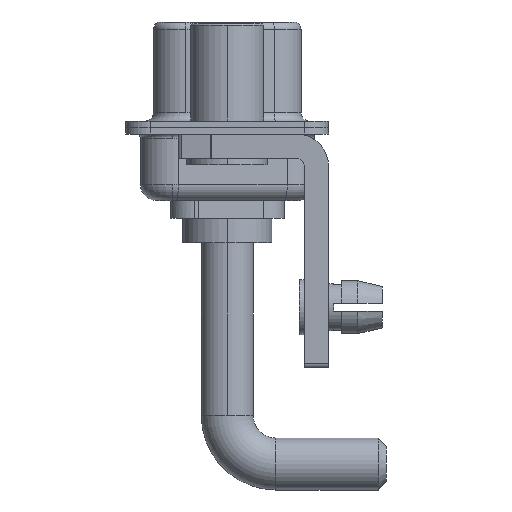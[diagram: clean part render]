
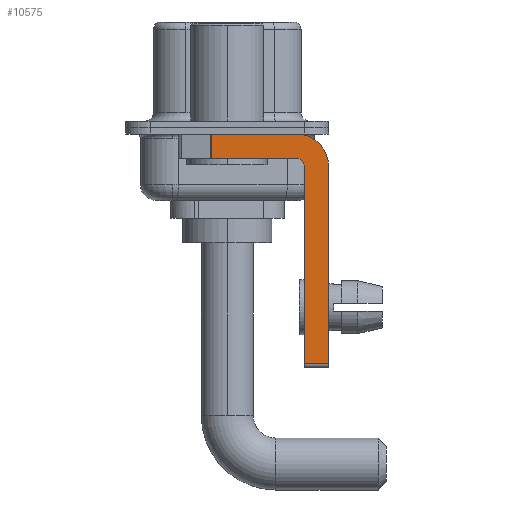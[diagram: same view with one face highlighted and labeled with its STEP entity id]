
A CAD part, left-side view. The second image highlights one B-rep face of the part: STEP entity #10575.
In plain terms, the highlighted planar face has unit normal (-1, 0, 0).
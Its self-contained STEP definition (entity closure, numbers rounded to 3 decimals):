
#59 = EDGE_CURVE ( 'NONE', #12031, #14969, #9710, .T. ) ;
#64 = LINE ( 'NONE', #1293, #7859 ) ;
#87 = DIRECTION ( 'NONE',  ( 0., 0., -1. ) ) ;
#227 = CARTESIAN_POINT ( 'NONE',  ( -2.9, -4.25, -2.4 ) ) ;
#367 = LINE ( 'NONE', #14322, #5056 ) ;
#567 = ORIENTED_EDGE ( 'NONE', *, *, #7969, .F. ) ;
#962 = CARTESIAN_POINT ( 'NONE',  ( -2.9, 0.978, -1.9 ) ) ;
#1140 = LINE ( 'NONE', #5623, #3806 ) ;
#1225 = ORIENTED_EDGE ( 'NONE', *, *, #59, .F. ) ;
#1293 = CARTESIAN_POINT ( 'NONE',  ( -2.9, -4.25, -1.9 ) ) ;
#1363 = AXIS2_PLACEMENT_3D ( 'NONE', #10004, #12916, #87 ) ;
#2270 = AXIS2_PLACEMENT_3D ( 'NONE', #227, #7632, #14753 ) ;
#2419 = DIRECTION ( 'NONE',  ( 0., -1., 0. ) ) ;
#2508 = AXIS2_PLACEMENT_3D ( 'NONE', #17097, #5567, #17004 ) ;
#3209 = EDGE_LOOP ( 'NONE', ( #5972, #3287, #11940, #4179, #567, #16561, #3625, #1225 ) ) ;
#3237 = EDGE_CURVE ( 'NONE', #15187, #3363, #10871, .T. ) ;
#3287 = ORIENTED_EDGE ( 'NONE', *, *, #15497, .T. ) ;
#3363 = VERTEX_POINT ( 'NONE', #15777 ) ;
#3625 = ORIENTED_EDGE ( 'NONE', *, *, #16791, .F. ) ;
#3655 = CARTESIAN_POINT ( 'NONE',  ( -2.9, 3., -0.4 ) ) ;
#3806 = VECTOR ( 'NONE', #9636, 1000. ) ;
#4096 = FACE_OUTER_BOUND ( 'NONE', #3209, .T. ) ;
#4100 = EDGE_CURVE ( 'NONE', #10009, #17103, #15181, .T. ) ;
#4179 = ORIENTED_EDGE ( 'NONE', *, *, #3237, .F. ) ;
#4200 = DIRECTION ( 'NONE',  ( 0., 1., 0. ) ) ;
#4389 = VECTOR ( 'NONE', #2419, 1000. ) ;
#5056 = VECTOR ( 'NONE', #6080, 1000. ) ;
#5198 = EDGE_CURVE ( 'NONE', #3363, #13883, #64, .T. ) ;
#5567 = DIRECTION ( 'NONE',  ( -1., 0., 0. ) ) ;
#5623 = CARTESIAN_POINT ( 'NONE',  ( -2.9, -4.75, -14.8 ) ) ;
#5701 = CARTESIAN_POINT ( 'NONE',  ( -2.9, -4.75, -14.55 ) ) ;
#5715 = LINE ( 'NONE', #18471, #17970 ) ;
#5972 = ORIENTED_EDGE ( 'NONE', *, *, #11311, .F. ) ;
#6080 = DIRECTION ( 'NONE',  ( 0., 0., -1. ) ) ;
#7314 = CARTESIAN_POINT ( 'NONE',  ( -2.9, -6.25, -2.4 ) ) ;
#7632 = DIRECTION ( 'NONE',  ( 1., 0., 0. ) ) ;
#7859 = VECTOR ( 'NONE', #4200, 1000. ) ;
#7969 = EDGE_CURVE ( 'NONE', #10009, #15187, #1140, .T. ) ;
#9439 = VERTEX_POINT ( 'NONE', #12837 ) ;
#9628 = LINE ( 'NONE', #3655, #4389 ) ;
#9636 = DIRECTION ( 'NONE',  ( 0., 0., 1. ) ) ;
#9710 = CIRCLE ( 'NONE', #1363, 2. ) ;
#9732 = DIRECTION ( 'NONE',  ( 0., 0., -1. ) ) ;
#9786 = PLANE ( 'NONE',  #2270 ) ;
#10004 = CARTESIAN_POINT ( 'NONE',  ( -2.9, -4.25, -2.4 ) ) ;
#10009 = VERTEX_POINT ( 'NONE', #5701 ) ;
#10575 = ADVANCED_FACE ( 'NONE', ( #4096 ), #9786, .F. ) ;
#10576 = CARTESIAN_POINT ( 'NONE',  ( -2.9, -4.75, -2.4 ) ) ;
#10871 = CIRCLE ( 'NONE', #2508, 0.5 ) ;
#11311 = EDGE_CURVE ( 'NONE', #9439, #12031, #9628, .T. ) ;
#11940 = ORIENTED_EDGE ( 'NONE', *, *, #5198, .F. ) ;
#12031 = VERTEX_POINT ( 'NONE', #16276 ) ;
#12837 = CARTESIAN_POINT ( 'NONE',  ( -2.9, 0.978, -0.4 ) ) ;
#12916 = DIRECTION ( 'NONE',  ( 1., 0., 0. ) ) ;
#13341 = VECTOR ( 'NONE', #13764, 1000. ) ;
#13764 = DIRECTION ( 'NONE',  ( 0., -1., 0. ) ) ;
#13883 = VERTEX_POINT ( 'NONE', #962 ) ;
#14322 = CARTESIAN_POINT ( 'NONE',  ( -2.9, 0.978, -1.9 ) ) ;
#14753 = DIRECTION ( 'NONE',  ( 0., 0., -1. ) ) ;
#14969 = VERTEX_POINT ( 'NONE', #7314 ) ;
#15181 = LINE ( 'NONE', #18087, #13341 ) ;
#15187 = VERTEX_POINT ( 'NONE', #10576 ) ;
#15497 = EDGE_CURVE ( 'NONE', #9439, #13883, #367, .T. ) ;
#15777 = CARTESIAN_POINT ( 'NONE',  ( -2.9, -4.25, -1.9 ) ) ;
#16276 = CARTESIAN_POINT ( 'NONE',  ( -2.9, -4.25, -0.4 ) ) ;
#16561 = ORIENTED_EDGE ( 'NONE', *, *, #4100, .T. ) ;
#16593 = CARTESIAN_POINT ( 'NONE',  ( -2.9, -6.25, -14.55 ) ) ;
#16791 = EDGE_CURVE ( 'NONE', #14969, #17103, #5715, .T. ) ;
#17004 = DIRECTION ( 'NONE',  ( 0., 0., 1. ) ) ;
#17097 = CARTESIAN_POINT ( 'NONE',  ( -2.9, -4.25, -2.4 ) ) ;
#17103 = VERTEX_POINT ( 'NONE', #16593 ) ;
#17970 = VECTOR ( 'NONE', #9732, 1000. ) ;
#18087 = CARTESIAN_POINT ( 'NONE',  ( -2.9, -4.25, -14.55 ) ) ;
#18471 = CARTESIAN_POINT ( 'NONE',  ( -2.9, -6.25, -2.4 ) ) ;
